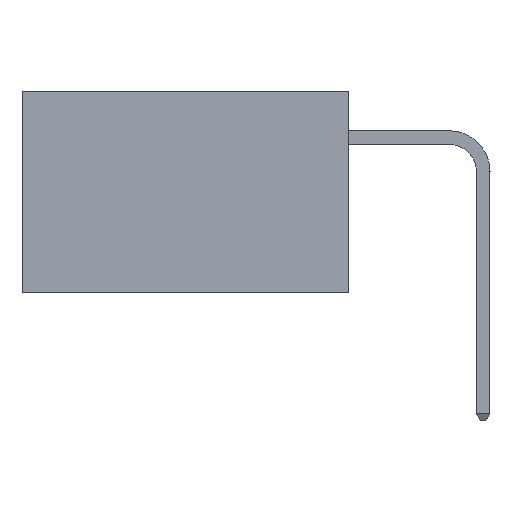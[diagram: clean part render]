
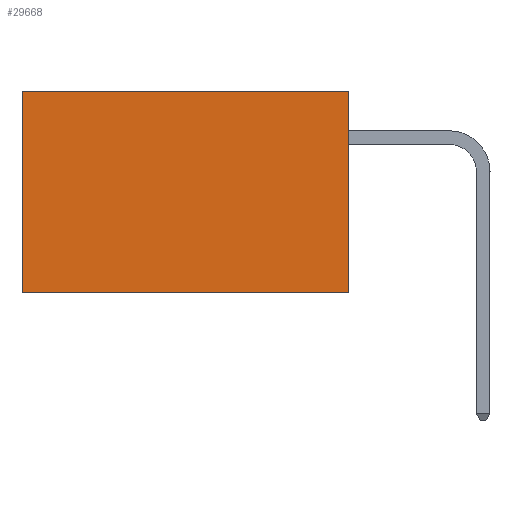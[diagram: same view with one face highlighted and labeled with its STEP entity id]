
A CAD part, left-side view. The second image highlights one B-rep face of the part: STEP entity #29668.
In plain terms, the highlighted planar face has unit normal (-1, 0, 0).
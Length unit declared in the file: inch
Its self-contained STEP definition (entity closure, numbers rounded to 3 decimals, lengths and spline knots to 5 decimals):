
#746 = DIRECTION ( 'NONE',  ( 0., 1., 0. ) ) ;
#1404 = VERTEX_POINT ( 'NONE', #22939 ) ;
#1957 = CARTESIAN_POINT ( 'NONE',  ( 0.2875, 0., -0.37 ) ) ;
#2603 = ORIENTED_EDGE ( 'NONE', *, *, #7163, .T. ) ;
#5083 = VECTOR ( 'NONE', #10577, 39.37008 ) ;
#5680 = VERTEX_POINT ( 'NONE', #21240 ) ;
#6714 = VECTOR ( 'NONE', #34322, 39.37008 ) ;
#6875 = FACE_OUTER_BOUND ( 'NONE', #18135, .T. ) ;
#7163 = EDGE_CURVE ( 'NONE', #34162, #1404, #15055, .T. ) ;
#7368 = VECTOR ( 'NONE', #28255, 39.37008 ) ;
#7445 = AXIS2_PLACEMENT_3D ( 'NONE', #16018, #7710, #26977 ) ;
#7710 = DIRECTION ( 'NONE',  ( 1., 0., 0. ) ) ;
#9481 = EDGE_CURVE ( 'NONE', #20304, #34162, #13068, .T. ) ;
#9908 = PLANE ( 'NONE',  #7445 ) ;
#10577 = DIRECTION ( 'NONE',  ( 0., 1., 0. ) ) ;
#12511 = LINE ( 'NONE', #1957, #5083 ) ;
#13068 = LINE ( 'NONE', #34057, #33899 ) ;
#14802 = LINE ( 'NONE', #17328, #7368 ) ;
#15055 = LINE ( 'NONE', #18153, #6714 ) ;
#16018 = CARTESIAN_POINT ( 'NONE',  ( 0.2875, 0., 0. ) ) ;
#16873 = EDGE_CURVE ( 'NONE', #5680, #1404, #12511, .T. ) ;
#17328 = CARTESIAN_POINT ( 'NONE',  ( 0.2875, 0., 0. ) ) ;
#18135 = EDGE_LOOP ( 'NONE', ( #2603, #27239, #28788, #27361 ) ) ;
#18153 = CARTESIAN_POINT ( 'NONE',  ( 0.2875, 0.6, 0. ) ) ;
#20304 = VERTEX_POINT ( 'NONE', #27522 ) ;
#21240 = CARTESIAN_POINT ( 'NONE',  ( 0.2875, 0., -0.37 ) ) ;
#22079 = CARTESIAN_POINT ( 'NONE',  ( 0.2875, 0.6, 0. ) ) ;
#22939 = CARTESIAN_POINT ( 'NONE',  ( 0.2875, 0.6, -0.37 ) ) ;
#25535 = EDGE_CURVE ( 'NONE', #20304, #5680, #14802, .T. ) ;
#26977 = DIRECTION ( 'NONE',  ( 0., 0., -1. ) ) ;
#27239 = ORIENTED_EDGE ( 'NONE', *, *, #16873, .F. ) ;
#27361 = ORIENTED_EDGE ( 'NONE', *, *, #9481, .T. ) ;
#27522 = CARTESIAN_POINT ( 'NONE',  ( 0.2875, 0., 0. ) ) ;
#28255 = DIRECTION ( 'NONE',  ( 0., 0., -1. ) ) ;
#28788 = ORIENTED_EDGE ( 'NONE', *, *, #25535, .F. ) ;
#29668 = ADVANCED_FACE ( 'NONE', ( #6875 ), #9908, .F. ) ;
#33899 = VECTOR ( 'NONE', #746, 39.37008 ) ;
#34057 = CARTESIAN_POINT ( 'NONE',  ( 0.2875, 0., 0. ) ) ;
#34162 = VERTEX_POINT ( 'NONE', #22079 ) ;
#34322 = DIRECTION ( 'NONE',  ( 0., 0., -1. ) ) ;
